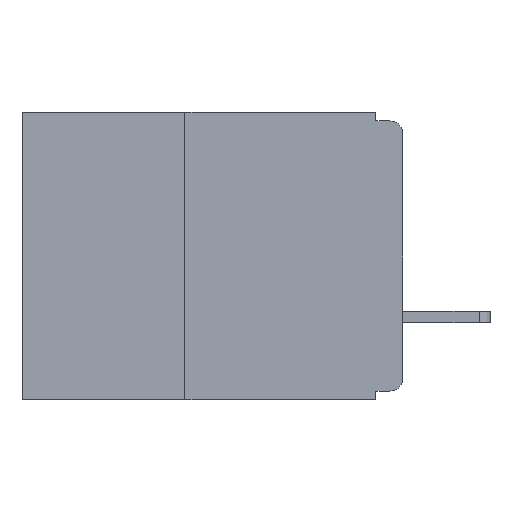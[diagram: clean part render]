
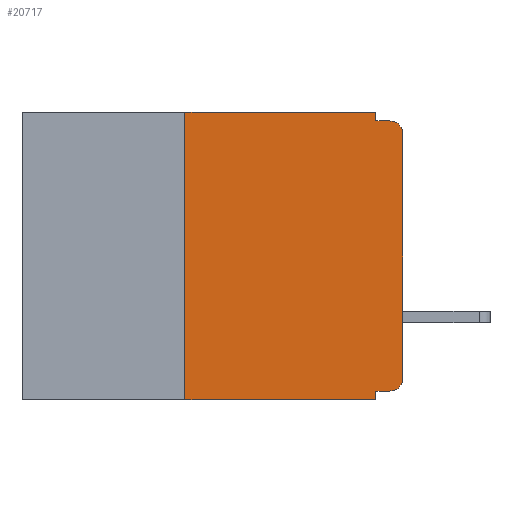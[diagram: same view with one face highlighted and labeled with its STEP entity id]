
A CAD part, left-side view. The second image highlights one B-rep face of the part: STEP entity #20717.
In plain terms, the highlighted planar face has unit normal (-1, 0, 0).
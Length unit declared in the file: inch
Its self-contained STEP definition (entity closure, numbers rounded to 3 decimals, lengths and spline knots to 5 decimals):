
#200 = ORIENTED_EDGE ( 'NONE', *, *, #24814, .F. ) ;
#216 = CARTESIAN_POINT ( 'NONE',  ( 0., 0.437, -0.33 ) ) ;
#306 = DIRECTION ( 'NONE',  ( 0., -1., 0. ) ) ;
#1203 = LINE ( 'NONE', #9163, #10660 ) ;
#1367 = VERTEX_POINT ( 'NONE', #25470 ) ;
#1699 = FACE_OUTER_BOUND ( 'NONE', #25296, .T. ) ;
#1841 = EDGE_CURVE ( 'NONE', #24717, #1914, #6849, .T. ) ;
#1914 = VERTEX_POINT ( 'NONE', #9661 ) ;
#2195 = EDGE_CURVE ( 'NONE', #14602, #6382, #23929, .T. ) ;
#3067 = PLANE ( 'NONE',  #25667 ) ;
#3349 = VECTOR ( 'NONE', #19516, 39.37008 ) ;
#3426 = ORIENTED_EDGE ( 'NONE', *, *, #4056, .F. ) ;
#3554 = VECTOR ( 'NONE', #306, 39.37008 ) ;
#3953 = CIRCLE ( 'NONE', #8211, 0.015 ) ;
#4054 = CARTESIAN_POINT ( 'NONE',  ( 0., 0.25, -0.33 ) ) ;
#4056 = EDGE_CURVE ( 'NONE', #24717, #6975, #15849, .T. ) ;
#4070 = VECTOR ( 'NONE', #22352, 39.37008 ) ;
#4079 = VERTEX_POINT ( 'NONE', #10092 ) ;
#4322 = EDGE_CURVE ( 'NONE', #4079, #22570, #14301, .T. ) ;
#4725 = CARTESIAN_POINT ( 'NONE',  ( 0., 0.015, -0.305 ) ) ;
#5981 = EDGE_CURVE ( 'NONE', #18117, #12918, #11704, .T. ) ;
#6236 = DIRECTION ( 'NONE',  ( -1., 0., 0. ) ) ;
#6382 = VERTEX_POINT ( 'NONE', #15683 ) ;
#6512 = CARTESIAN_POINT ( 'NONE',  ( 0., 0.015, -0.025 ) ) ;
#6849 = CIRCLE ( 'NONE', #9221, 0.015 ) ;
#6975 = VERTEX_POINT ( 'NONE', #23722 ) ;
#7113 = EDGE_CURVE ( 'NONE', #1914, #1367, #9439, .T. ) ;
#7212 = DIRECTION ( 'NONE',  ( 0., 0., -1. ) ) ;
#8211 = AXIS2_PLACEMENT_3D ( 'NONE', #6512, #20464, #8534 ) ;
#8376 = EDGE_CURVE ( 'NONE', #4079, #18117, #10007, .T. ) ;
#8405 = DIRECTION ( 'NONE',  ( 0., -1., 0. ) ) ;
#8419 = ORIENTED_EDGE ( 'NONE', *, *, #24334, .F. ) ;
#8534 = DIRECTION ( 'NONE',  ( 0., 0., -1. ) ) ;
#9163 = CARTESIAN_POINT ( 'NONE',  ( 0., 0.031, 0. ) ) ;
#9175 = DIRECTION ( 'NONE',  ( 0., 0., -1. ) ) ;
#9221 = AXIS2_PLACEMENT_3D ( 'NONE', #4725, #6236, #23489 ) ;
#9439 = LINE ( 'NONE', #16416, #4070 ) ;
#9661 = CARTESIAN_POINT ( 'NONE',  ( 0., 0., -0.305 ) ) ;
#9970 = CARTESIAN_POINT ( 'NONE',  ( 0., 0.031, 0. ) ) ;
#10007 = LINE ( 'NONE', #4054, #20566 ) ;
#10026 = ORIENTED_EDGE ( 'NONE', *, *, #8376, .F. ) ;
#10092 = CARTESIAN_POINT ( 'NONE',  ( 0., 0.25, -0.33 ) ) ;
#10427 = CARTESIAN_POINT ( 'NONE',  ( 0., 0.437, 0. ) ) ;
#10660 = VECTOR ( 'NONE', #7212, 39.37008 ) ;
#10879 = CARTESIAN_POINT ( 'NONE',  ( 0., 0.015, -0.32 ) ) ;
#10896 = DIRECTION ( 'NONE',  ( 0., 1., 0. ) ) ;
#11156 = CARTESIAN_POINT ( 'NONE',  ( 0., 0., -0.32 ) ) ;
#11572 = ORIENTED_EDGE ( 'NONE', *, *, #5981, .F. ) ;
#11704 = LINE ( 'NONE', #10427, #21621 ) ;
#12852 = ORIENTED_EDGE ( 'NONE', *, *, #19298, .T. ) ;
#12918 = VERTEX_POINT ( 'NONE', #9970 ) ;
#13215 = DIRECTION ( 'NONE',  ( 0., 0., -1. ) ) ;
#13492 = VECTOR ( 'NONE', #13215, 39.37008 ) ;
#14301 = LINE ( 'NONE', #216, #3554 ) ;
#14602 = VERTEX_POINT ( 'NONE', #24730 ) ;
#14998 = CARTESIAN_POINT ( 'NONE',  ( 0., 0.25, 0. ) ) ;
#15019 = ORIENTED_EDGE ( 'NONE', *, *, #7113, .T. ) ;
#15206 = CARTESIAN_POINT ( 'NONE',  ( 0., 0.031, -0.33 ) ) ;
#15683 = CARTESIAN_POINT ( 'NONE',  ( 0., 0.015, -0.01 ) ) ;
#15849 = LINE ( 'NONE', #11156, #25651 ) ;
#16089 = DIRECTION ( 'NONE',  ( 0., 0., 1. ) ) ;
#16416 = CARTESIAN_POINT ( 'NONE',  ( 0., 0., 0. ) ) ;
#16974 = ORIENTED_EDGE ( 'NONE', *, *, #1841, .T. ) ;
#18117 = VERTEX_POINT ( 'NONE', #14998 ) ;
#19021 = CARTESIAN_POINT ( 'NONE',  ( 0., 0.437, 0. ) ) ;
#19298 = EDGE_CURVE ( 'NONE', #1367, #6382, #3953, .T. ) ;
#19318 = CARTESIAN_POINT ( 'NONE',  ( 0., 0., -0.01 ) ) ;
#19321 = ORIENTED_EDGE ( 'NONE', *, *, #2195, .F. ) ;
#19516 = DIRECTION ( 'NONE',  ( 0., -1., 0. ) ) ;
#20464 = DIRECTION ( 'NONE',  ( -1., 0., 0. ) ) ;
#20566 = VECTOR ( 'NONE', #16089, 39.37008 ) ;
#20717 = ADVANCED_FACE ( 'NONE', ( #1699 ), #3067, .F. ) ;
#21072 = DIRECTION ( 'NONE',  ( 1., 0., 0. ) ) ;
#21621 = VECTOR ( 'NONE', #8405, 39.37008 ) ;
#22352 = DIRECTION ( 'NONE',  ( 0., 0., 1. ) ) ;
#22570 = VERTEX_POINT ( 'NONE', #24958 ) ;
#23341 = LINE ( 'NONE', #15206, #13492 ) ;
#23489 = DIRECTION ( 'NONE',  ( 0., 0., -1. ) ) ;
#23722 = CARTESIAN_POINT ( 'NONE',  ( 0., 0.031, -0.32 ) ) ;
#23929 = LINE ( 'NONE', #19318, #3349 ) ;
#24334 = EDGE_CURVE ( 'NONE', #12918, #14602, #1203, .T. ) ;
#24717 = VERTEX_POINT ( 'NONE', #10879 ) ;
#24730 = CARTESIAN_POINT ( 'NONE',  ( 0., 0.031, -0.01 ) ) ;
#24814 = EDGE_CURVE ( 'NONE', #6975, #22570, #23341, .T. ) ;
#24876 = ORIENTED_EDGE ( 'NONE', *, *, #4322, .T. ) ;
#24958 = CARTESIAN_POINT ( 'NONE',  ( 0., 0.031, -0.33 ) ) ;
#25296 = EDGE_LOOP ( 'NONE', ( #15019, #12852, #19321, #8419, #11572, #10026, #24876, #200, #3426, #16974 ) ) ;
#25470 = CARTESIAN_POINT ( 'NONE',  ( 0., 0., -0.025 ) ) ;
#25651 = VECTOR ( 'NONE', #10896, 39.37008 ) ;
#25667 = AXIS2_PLACEMENT_3D ( 'NONE', #19021, #21072, #9175 ) ;
